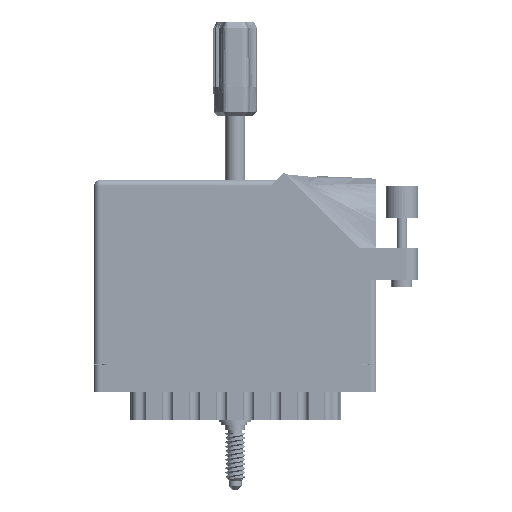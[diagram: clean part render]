
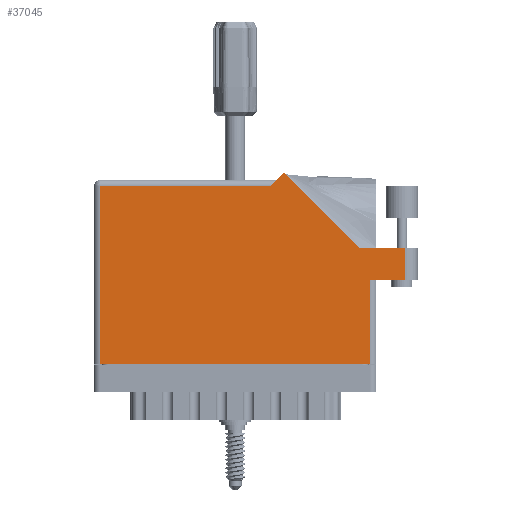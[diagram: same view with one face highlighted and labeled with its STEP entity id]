
A CAD part, front view. The second image highlights one B-rep face of the part: STEP entity #37045.
In plain terms, the highlighted face is planar.
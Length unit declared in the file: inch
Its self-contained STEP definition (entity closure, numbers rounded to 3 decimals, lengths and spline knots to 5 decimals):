
#1005 = CARTESIAN_POINT ( 'NONE',  ( 0., 1.713, 0. ) ) ;
#2046 = EDGE_LOOP ( 'NONE', ( #30069, #73817, #39880, #82738, #13847, #3331, #78158, #29232, #76976 ) ) ;
#3120 = CARTESIAN_POINT ( 'NONE',  ( 0., 0., 0. ) ) ;
#3331 = ORIENTED_EDGE ( 'NONE', *, *, #42883, .T. ) ;
#5730 = DIRECTION ( 'NONE',  ( 0., 0., -1. ) ) ;
#6389 = CARTESIAN_POINT ( 'NONE',  ( 2.993, 1.122, 0. ) ) ;
#6917 = CARTESIAN_POINT ( 'NONE',  ( 1.82871, 1.84571, 0. ) ) ;
#7416 = CARTESIAN_POINT ( 'NONE',  ( 2.993, 0.815, 0. ) ) ;
#10676 = CARTESIAN_POINT ( 'NONE',  ( 2.55242, 1.122, 0. ) ) ;
#11454 = CARTESIAN_POINT ( 'NONE',  ( 2.55242, 1.122, 0. ) ) ;
#13338 = EDGE_CURVE ( 'NONE', #74434, #14721, #21533, .T. ) ;
#13808 = DIRECTION ( 'NONE',  ( 1., 0., 0. ) ) ;
#13847 = ORIENTED_EDGE ( 'NONE', *, *, #80242, .T. ) ;
#14305 = DIRECTION ( 'NONE',  ( -1., 0., 0. ) ) ;
#14387 = CARTESIAN_POINT ( 'NONE',  ( 2.718, 0.815, 0. ) ) ;
#14721 = VERTEX_POINT ( 'NONE', #38168 ) ;
#14724 = LINE ( 'NONE', #10676, #47211 ) ;
#15221 = EDGE_CURVE ( 'NONE', #46657, #71242, #14724, .T. ) ;
#17513 = VECTOR ( 'NONE', #39620, 39.37008 ) ;
#20954 = VECTOR ( 'NONE', #57625, 39.37008 ) ;
#21533 = LINE ( 'NONE', #87993, #34577 ) ;
#25700 = VERTEX_POINT ( 'NONE', #6389 ) ;
#26884 = CARTESIAN_POINT ( 'NONE',  ( 2.993, 1.122, 0. ) ) ;
#27241 = FACE_OUTER_BOUND ( 'NONE', #2046, .T. ) ;
#29232 = ORIENTED_EDGE ( 'NONE', *, *, #75828, .T. ) ;
#30069 = ORIENTED_EDGE ( 'NONE', *, *, #47292, .T. ) ;
#30259 = LINE ( 'NONE', #1005, #46489 ) ;
#30541 = LINE ( 'NONE', #14387, #74842 ) ;
#32683 = LINE ( 'NONE', #76711, #62938 ) ;
#34450 = DIRECTION ( 'NONE',  ( 0., 1., 0. ) ) ;
#34577 = VECTOR ( 'NONE', #44202, 39.37008 ) ;
#35349 = DIRECTION ( 'NONE',  ( 0., 1., 0. ) ) ;
#35924 = VECTOR ( 'NONE', #34450, 39.37008 ) ;
#37045 = ADVANCED_FACE ( 'NONE', ( #27241 ), #68291, .F. ) ;
#37164 = CARTESIAN_POINT ( 'NONE',  ( 2.656, 0.815, 0. ) ) ;
#38168 = CARTESIAN_POINT ( 'NONE',  ( 0.062, 0., 0. ) ) ;
#38545 = DIRECTION ( 'NONE',  ( -0.707, 0.707, 0. ) ) ;
#39620 = DIRECTION ( 'NONE',  ( -1., 0., 0. ) ) ;
#39880 = ORIENTED_EDGE ( 'NONE', *, *, #47174, .T. ) ;
#40799 = CARTESIAN_POINT ( 'NONE',  ( 3.118, 1.122, 0. ) ) ;
#41424 = DIRECTION ( 'NONE',  ( -1., 0., 0. ) ) ;
#42883 = EDGE_CURVE ( 'NONE', #89333, #74434, #30259, .T. ) ;
#43591 = CARTESIAN_POINT ( 'NONE',  ( 1.696, 1.713, 0. ) ) ;
#44202 = DIRECTION ( 'NONE',  ( 0., -1., 0. ) ) ;
#45046 = LINE ( 'NONE', #82753, #48320 ) ;
#46489 = VECTOR ( 'NONE', #14305, 39.37008 ) ;
#46657 = VERTEX_POINT ( 'NONE', #11454 ) ;
#46932 = CARTESIAN_POINT ( 'NONE',  ( 2.656, 0., 0. ) ) ;
#47174 = EDGE_CURVE ( 'NONE', #25700, #46657, #71603, .T. ) ;
#47211 = VECTOR ( 'NONE', #38545, 39.37008 ) ;
#47292 = EDGE_CURVE ( 'NONE', #67322, #82450, #30541, .T. ) ;
#48320 = VECTOR ( 'NONE', #55285, 39.37008 ) ;
#54330 = LINE ( 'NONE', #26884, #35924 ) ;
#55285 = DIRECTION ( 'NONE',  ( -0.707, -0.707, 0. ) ) ;
#57625 = DIRECTION ( 'NONE',  ( 1., 0., 0. ) ) ;
#62938 = VECTOR ( 'NONE', #35349, 39.37008 ) ;
#65273 = LINE ( 'NONE', #3120, #20954 ) ;
#67322 = VERTEX_POINT ( 'NONE', #37164 ) ;
#68291 = PLANE ( 'NONE',  #82927 ) ;
#69833 = CARTESIAN_POINT ( 'NONE',  ( 0.062, 1.713, 0. ) ) ;
#71219 = EDGE_CURVE ( 'NONE', #82450, #25700, #54330, .T. ) ;
#71242 = VERTEX_POINT ( 'NONE', #6917 ) ;
#71603 = LINE ( 'NONE', #40799, #17513 ) ;
#73817 = ORIENTED_EDGE ( 'NONE', *, *, #71219, .T. ) ;
#74434 = VERTEX_POINT ( 'NONE', #69833 ) ;
#74842 = VECTOR ( 'NONE', #13808, 39.37008 ) ;
#75828 = EDGE_CURVE ( 'NONE', #14721, #81154, #65273, .T. ) ;
#76711 = CARTESIAN_POINT ( 'NONE',  ( 2.656, 0.815, 0. ) ) ;
#76976 = ORIENTED_EDGE ( 'NONE', *, *, #87671, .T. ) ;
#78158 = ORIENTED_EDGE ( 'NONE', *, *, #13338, .T. ) ;
#80242 = EDGE_CURVE ( 'NONE', #71242, #89333, #45046, .T. ) ;
#81154 = VERTEX_POINT ( 'NONE', #46932 ) ;
#82450 = VERTEX_POINT ( 'NONE', #7416 ) ;
#82738 = ORIENTED_EDGE ( 'NONE', *, *, #15221, .T. ) ;
#82753 = CARTESIAN_POINT ( 'NONE',  ( 1.758, 1.775, 0. ) ) ;
#82779 = CARTESIAN_POINT ( 'NONE',  ( 0., 1.775, 0. ) ) ;
#82927 = AXIS2_PLACEMENT_3D ( 'NONE', #82779, #5730, #41424 ) ;
#87671 = EDGE_CURVE ( 'NONE', #81154, #67322, #32683, .T. ) ;
#87993 = CARTESIAN_POINT ( 'NONE',  ( 0.062, 0., 0. ) ) ;
#89333 = VERTEX_POINT ( 'NONE', #43591 ) ;
